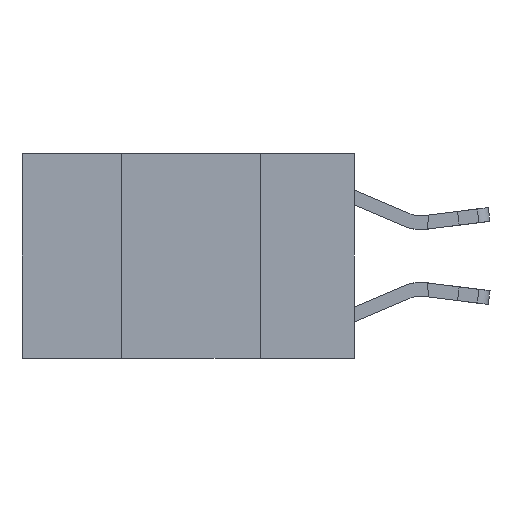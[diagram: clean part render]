
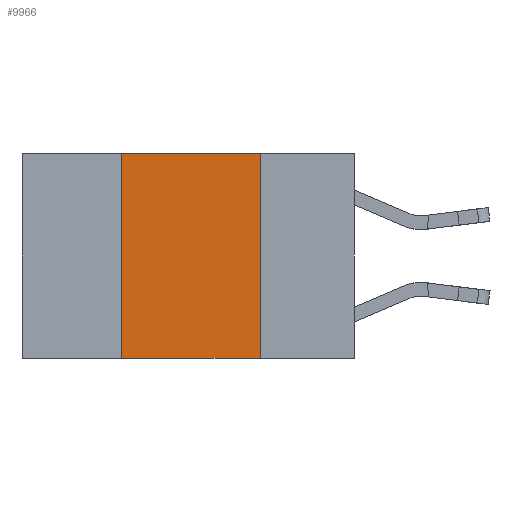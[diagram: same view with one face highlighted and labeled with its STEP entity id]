
A CAD part, left-side view. The second image highlights one B-rep face of the part: STEP entity #9966.
In plain terms, the highlighted planar face has unit normal (-1, 0, 0).
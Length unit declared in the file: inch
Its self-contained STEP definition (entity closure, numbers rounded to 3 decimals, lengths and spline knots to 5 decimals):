
#792 = DIRECTION ( 'NONE',  ( 0., -1., 0. ) ) ;
#1239 = LINE ( 'NONE', #11292, #14532 ) ;
#1902 = LINE ( 'NONE', #15345, #8560 ) ;
#2042 = EDGE_CURVE ( 'NONE', #6432, #9509, #1902, .T. ) ;
#2587 = LINE ( 'NONE', #8905, #9252 ) ;
#3115 = VERTEX_POINT ( 'NONE', #13413 ) ;
#3843 = ORIENTED_EDGE ( 'NONE', *, *, #2042, .F. ) ;
#4261 = ORIENTED_EDGE ( 'NONE', *, *, #14733, .F. ) ;
#4665 = ORIENTED_EDGE ( 'NONE', *, *, #11110, .T. ) ;
#6348 = PLANE ( 'NONE',  #9453 ) ;
#6432 = VERTEX_POINT ( 'NONE', #8111 ) ;
#6544 = ORIENTED_EDGE ( 'NONE', *, *, #14731, .F. ) ;
#7697 = DIRECTION ( 'NONE',  ( 1., 0., 0. ) ) ;
#8111 = CARTESIAN_POINT ( 'NONE',  ( 0., 0.42, 0. ) ) ;
#8560 = VECTOR ( 'NONE', #792, 39.37008 ) ;
#8905 = CARTESIAN_POINT ( 'NONE',  ( 0., 0.42, 0. ) ) ;
#9252 = VECTOR ( 'NONE', #10226, 39.37008 ) ;
#9453 = AXIS2_PLACEMENT_3D ( 'NONE', #15614, #7697, #16939 ) ;
#9509 = VERTEX_POINT ( 'NONE', #13180 ) ;
#9658 = LINE ( 'NONE', #15502, #16267 ) ;
#9966 = ADVANCED_FACE ( 'NONE', ( #15011 ), #6348, .F. ) ;
#10210 = CARTESIAN_POINT ( 'NONE',  ( 0., 0.42, -0.37 ) ) ;
#10226 = DIRECTION ( 'NONE',  ( 0., 0., 1. ) ) ;
#11110 = EDGE_CURVE ( 'NONE', #13368, #3115, #1239, .T. ) ;
#11292 = CARTESIAN_POINT ( 'NONE',  ( 0., 0.6, -0.37 ) ) ;
#13180 = CARTESIAN_POINT ( 'NONE',  ( 0., 0.17, 0. ) ) ;
#13368 = VERTEX_POINT ( 'NONE', #10210 ) ;
#13413 = CARTESIAN_POINT ( 'NONE',  ( 0., 0.17, -0.37 ) ) ;
#14532 = VECTOR ( 'NONE', #16608, 39.37008 ) ;
#14731 = EDGE_CURVE ( 'NONE', #9509, #3115, #9658, .T. ) ;
#14733 = EDGE_CURVE ( 'NONE', #13368, #6432, #2587, .T. ) ;
#15011 = FACE_OUTER_BOUND ( 'NONE', #16033, .T. ) ;
#15345 = CARTESIAN_POINT ( 'NONE',  ( 0., 0.6, 0. ) ) ;
#15502 = CARTESIAN_POINT ( 'NONE',  ( 0., 0.17, 0. ) ) ;
#15614 = CARTESIAN_POINT ( 'NONE',  ( 0., 0.6, 0. ) ) ;
#16033 = EDGE_LOOP ( 'NONE', ( #6544, #3843, #4261, #4665 ) ) ;
#16267 = VECTOR ( 'NONE', #16807, 39.37008 ) ;
#16608 = DIRECTION ( 'NONE',  ( 0., -1., 0. ) ) ;
#16807 = DIRECTION ( 'NONE',  ( 0., 0., -1. ) ) ;
#16939 = DIRECTION ( 'NONE',  ( 0., 0., -1. ) ) ;
